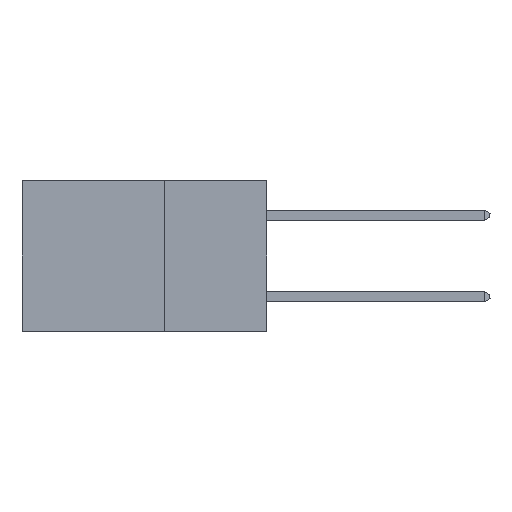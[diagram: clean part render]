
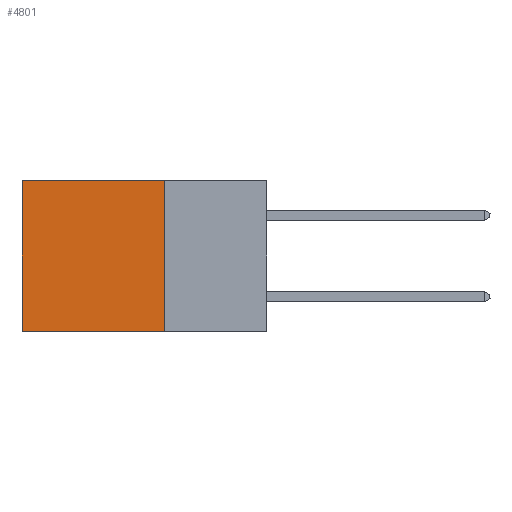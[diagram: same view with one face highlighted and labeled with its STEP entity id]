
A CAD part, left-side view. The second image highlights one B-rep face of the part: STEP entity #4801.
In plain terms, the highlighted planar face has unit normal (-1, 0, 0).
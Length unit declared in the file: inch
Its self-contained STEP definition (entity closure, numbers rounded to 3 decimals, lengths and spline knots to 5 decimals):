
#876 = CARTESIAN_POINT ( 'NONE',  ( 0.2875, 0.6, -0.37 ) ) ;
#1162 = VERTEX_POINT ( 'NONE', #876 ) ;
#1899 = VECTOR ( 'NONE', #10219, 39.37008 ) ;
#1983 = VECTOR ( 'NONE', #15769, 39.37008 ) ;
#2104 = PLANE ( 'NONE',  #16609 ) ;
#2562 = EDGE_CURVE ( 'NONE', #6479, #3311, #7934, .T. ) ;
#2675 = CARTESIAN_POINT ( 'NONE',  ( 0.2875, 0.6, 0. ) ) ;
#3311 = VERTEX_POINT ( 'NONE', #14582 ) ;
#4423 = FACE_OUTER_BOUND ( 'NONE', #7500, .T. ) ;
#4606 = CARTESIAN_POINT ( 'NONE',  ( 0.2875, 0.25, 0. ) ) ;
#4801 = ADVANCED_FACE ( 'NONE', ( #4423 ), #2104, .F. ) ;
#6479 = VERTEX_POINT ( 'NONE', #15717 ) ;
#6853 = LINE ( 'NONE', #18202, #1899 ) ;
#6877 = VECTOR ( 'NONE', #17606, 39.37008 ) ;
#7112 = LINE ( 'NONE', #7407, #19451 ) ;
#7407 = CARTESIAN_POINT ( 'NONE',  ( 0.2875, 0.25, 0. ) ) ;
#7466 = LINE ( 'NONE', #2675, #1983 ) ;
#7500 = EDGE_LOOP ( 'NONE', ( #8667, #12932, #13723, #12930 ) ) ;
#7755 = VERTEX_POINT ( 'NONE', #12664 ) ;
#7934 = LINE ( 'NONE', #4606, #6877 ) ;
#8667 = ORIENTED_EDGE ( 'NONE', *, *, #14503, .T. ) ;
#8846 = DIRECTION ( 'NONE',  ( 0., 0., -1. ) ) ;
#9772 = EDGE_CURVE ( 'NONE', #6479, #7755, #7112, .T. ) ;
#10219 = DIRECTION ( 'NONE',  ( 0., 1., 0. ) ) ;
#12664 = CARTESIAN_POINT ( 'NONE',  ( 0.2875, 0.6, 0. ) ) ;
#12930 = ORIENTED_EDGE ( 'NONE', *, *, #9772, .T. ) ;
#12932 = ORIENTED_EDGE ( 'NONE', *, *, #16172, .F. ) ;
#13723 = ORIENTED_EDGE ( 'NONE', *, *, #2562, .F. ) ;
#14503 = EDGE_CURVE ( 'NONE', #7755, #1162, #7466, .T. ) ;
#14582 = CARTESIAN_POINT ( 'NONE',  ( 0.2875, 0.25, -0.37 ) ) ;
#15243 = CARTESIAN_POINT ( 'NONE',  ( 0.2875, 0.25, 0. ) ) ;
#15717 = CARTESIAN_POINT ( 'NONE',  ( 0.2875, 0.25, 0. ) ) ;
#15769 = DIRECTION ( 'NONE',  ( 0., 0., -1. ) ) ;
#16172 = EDGE_CURVE ( 'NONE', #3311, #1162, #6853, .T. ) ;
#16609 = AXIS2_PLACEMENT_3D ( 'NONE', #15243, #18410, #8846 ) ;
#17606 = DIRECTION ( 'NONE',  ( 0., 0., -1. ) ) ;
#18202 = CARTESIAN_POINT ( 'NONE',  ( 0.2875, 0.25, -0.37 ) ) ;
#18410 = DIRECTION ( 'NONE',  ( 1., 0., 0. ) ) ;
#19451 = VECTOR ( 'NONE', #20258, 39.37008 ) ;
#20258 = DIRECTION ( 'NONE',  ( 0., 1., 0. ) ) ;
